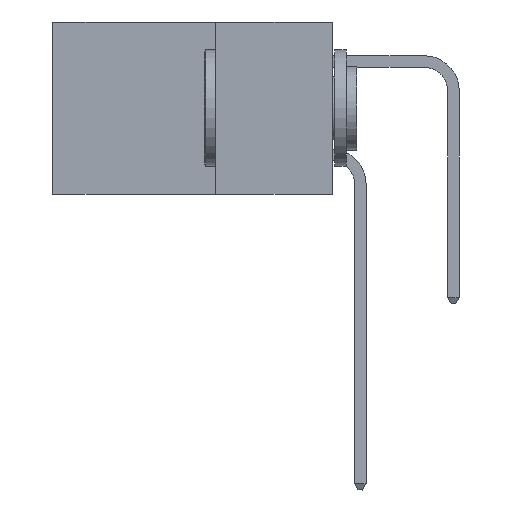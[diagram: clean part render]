
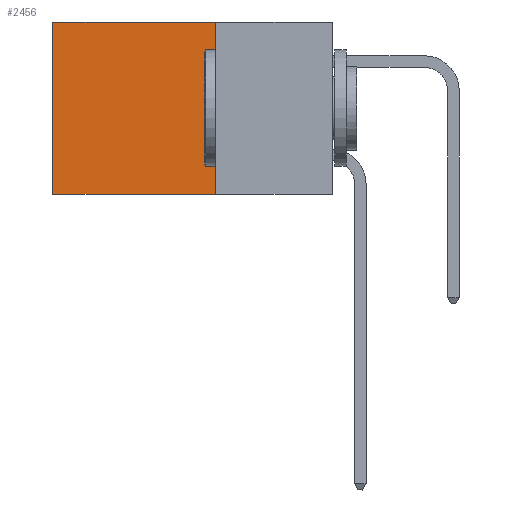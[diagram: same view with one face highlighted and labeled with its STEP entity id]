
A CAD part, left-side view. The second image highlights one B-rep face of the part: STEP entity #2456.
In plain terms, the highlighted planar face has unit normal (-1, 0, 0).
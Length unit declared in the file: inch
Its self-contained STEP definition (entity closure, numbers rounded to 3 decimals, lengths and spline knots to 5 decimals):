
#104 = DIRECTION ( 'NONE',  ( 0., 0., -1. ) ) ;
#588 = EDGE_LOOP ( 'NONE', ( #9900, #8659, #2035, #7698 ) ) ;
#671 = VECTOR ( 'NONE', #9387, 39.37008 ) ;
#874 = AXIS2_PLACEMENT_3D ( 'NONE', #5171, #3357, #4265 ) ;
#955 = LINE ( 'NONE', #7436, #671 ) ;
#1325 = EDGE_CURVE ( 'NONE', #7098, #8997, #8226, .T. ) ;
#1332 = VERTEX_POINT ( 'NONE', #6273 ) ;
#2035 = ORIENTED_EDGE ( 'NONE', *, *, #7532, .F. ) ;
#2082 = VECTOR ( 'NONE', #5423, 39.37008 ) ;
#2456 = ADVANCED_FACE ( 'NONE', ( #2529 ), #10728, .F. ) ;
#2529 = FACE_OUTER_BOUND ( 'NONE', #588, .T. ) ;
#3357 = DIRECTION ( 'NONE',  ( 1., 0., 0. ) ) ;
#4265 = DIRECTION ( 'NONE',  ( 0., 0., -1. ) ) ;
#5171 = CARTESIAN_POINT ( 'NONE',  ( 0.2615, 0.25, -0.37 ) ) ;
#5375 = CARTESIAN_POINT ( 'NONE',  ( 0.2615, 0.25, -0.37 ) ) ;
#5408 = EDGE_CURVE ( 'NONE', #1332, #7098, #955, .T. ) ;
#5423 = DIRECTION ( 'NONE',  ( 0., 1., 0. ) ) ;
#5978 = VECTOR ( 'NONE', #7311, 39.37008 ) ;
#6273 = CARTESIAN_POINT ( 'NONE',  ( 0.2615, 0.25, 0. ) ) ;
#7098 = VERTEX_POINT ( 'NONE', #8647 ) ;
#7305 = VECTOR ( 'NONE', #104, 39.37008 ) ;
#7311 = DIRECTION ( 'NONE',  ( 0., 0., -1. ) ) ;
#7436 = CARTESIAN_POINT ( 'NONE',  ( 0.2615, 0.25, 0. ) ) ;
#7532 = EDGE_CURVE ( 'NONE', #1332, #8750, #10192, .T. ) ;
#7698 = ORIENTED_EDGE ( 'NONE', *, *, #5408, .T. ) ;
#7755 = EDGE_CURVE ( 'NONE', #8750, #8997, #10917, .T. ) ;
#8226 = LINE ( 'NONE', #10924, #5978 ) ;
#8270 = CARTESIAN_POINT ( 'NONE',  ( 0.2615, 0.25, -0.37 ) ) ;
#8358 = CARTESIAN_POINT ( 'NONE',  ( 0.2615, 0.25, -0.37 ) ) ;
#8647 = CARTESIAN_POINT ( 'NONE',  ( 0.2615, 0.6, 0. ) ) ;
#8659 = ORIENTED_EDGE ( 'NONE', *, *, #7755, .F. ) ;
#8750 = VERTEX_POINT ( 'NONE', #5375 ) ;
#8997 = VERTEX_POINT ( 'NONE', #11706 ) ;
#9387 = DIRECTION ( 'NONE',  ( 0., 1., 0. ) ) ;
#9900 = ORIENTED_EDGE ( 'NONE', *, *, #1325, .T. ) ;
#10192 = LINE ( 'NONE', #8358, #7305 ) ;
#10728 = PLANE ( 'NONE',  #874 ) ;
#10917 = LINE ( 'NONE', #8270, #2082 ) ;
#10924 = CARTESIAN_POINT ( 'NONE',  ( 0.2615, 0.6, -0.37 ) ) ;
#11706 = CARTESIAN_POINT ( 'NONE',  ( 0.2615, 0.6, -0.37 ) ) ;
